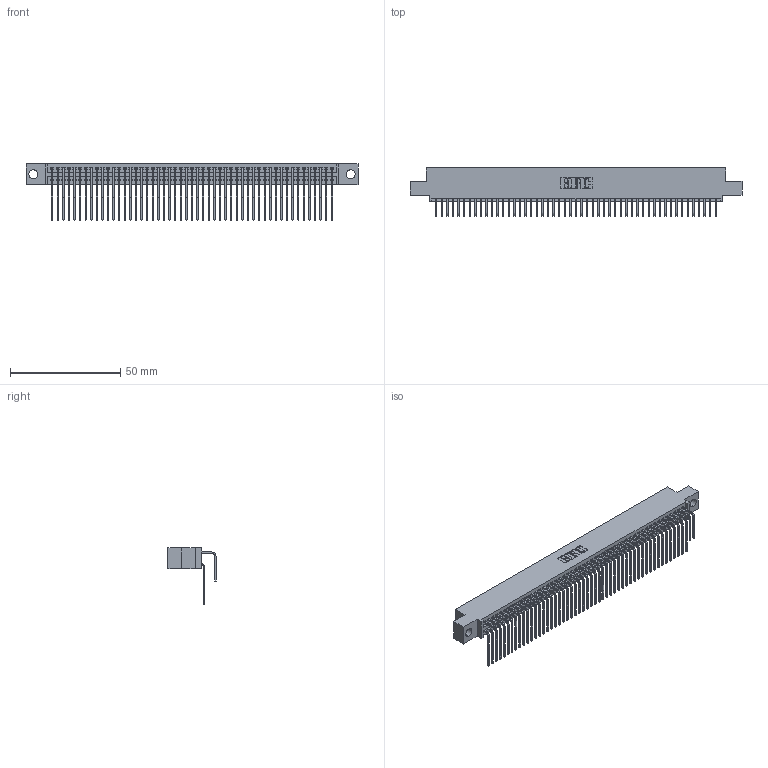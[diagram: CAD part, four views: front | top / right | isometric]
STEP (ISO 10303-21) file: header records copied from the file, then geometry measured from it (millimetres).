
FILE_DESCRIPTION (( 'STEP AP203' ), '1' );
FILE_NAME ('395-102-558-504.STEP', '2018-11-30T09:44:16', ( '' ), ( '' ), 'SwSTEP 2.0', 'SolidWorks 2016', '' );
FILE_SCHEMA (( 'CONFIG_CONTROL_DESIGN' ));
Length unit declared in the file: inch
Products named in the file (4): 345-292-001_558 559 Tail - 1; 345 Part_0.110 Offset - 0.156 Dia-TH; 395-102-558-504; 345-292-001_558 Tail - 2
Assembly tree (103 placements, depth 2):
  395-102-558-504
    345 Part_0.110 Offset - 0.156 Dia-TH
    345-292-001_558 559 Tail - 1  x51
    345-292-001_558 Tail - 2  x51
Bounding box: 150.75 x 21.83 x 25.53 mm (x, y, z)
Volume: 15154.6 mm3; surface area: 25250.3 mm2
Topology: 103 solids, 103 shells, 5434 faces, 16163 edges, 10638 vertices
Faces by surface type: plane 3654, cylinder 1780
Entity records: 40591 total; most frequent: CARTESIAN_POINT 6843, ORIENTED_EDGE 6726, DIRECTION 5995, EDGE_CURVE 3363, LINE 2987, VECTOR 2987, VERTEX_POINT 2238, AXIS2_PLACEMENT_3D 1504
